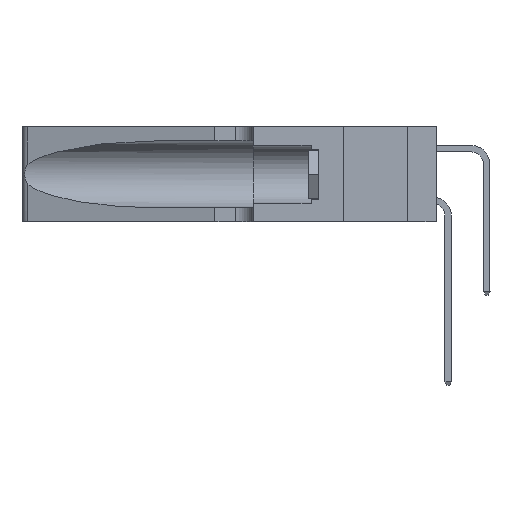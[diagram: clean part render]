
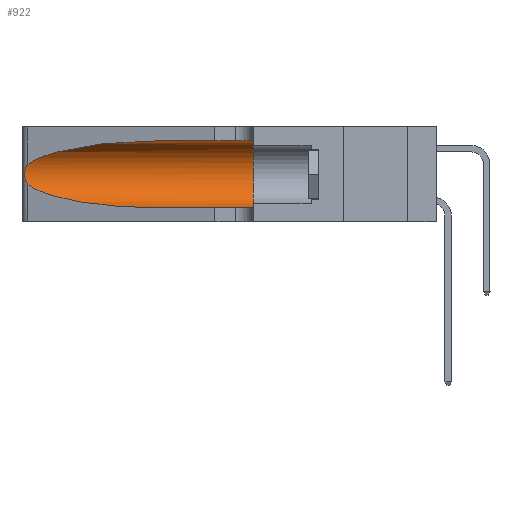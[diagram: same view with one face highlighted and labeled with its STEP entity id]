
A CAD part, left-side view. The second image highlights one B-rep face of the part: STEP entity #922.
In plain terms, the highlighted cylindrical face has radius 3.308 mm (diameter 6.617 mm), a partial arc.
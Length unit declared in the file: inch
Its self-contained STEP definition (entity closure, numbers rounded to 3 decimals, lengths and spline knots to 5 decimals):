
#922 = ADVANCED_FACE ( 'NONE', ( #21679 ), #20278, .F. ) ;
#975 = CARTESIAN_POINT ( 'NONE',  ( 0.25487, 1.22718, 0.14631 ) ) ;
#1325 = AXIS2_PLACEMENT_3D ( 'NONE', #26739, #13287, #20178 ) ;
#2145 = ORIENTED_EDGE ( 'NONE', *, *, #12328, .F. ) ;
#2264 = LINE ( 'NONE', #24805, #27629 ) ;
#3029 = VERTEX_POINT ( 'NONE', #3375 ) ;
#3375 = CARTESIAN_POINT ( 'NONE',  ( 0.1305, 0.35, 0.05475 ) ) ;
#4745 = CARTESIAN_POINT ( 'NONE',  ( 0.25555, 1.22994, 0.2215 ) ) ;
#5323 = CARTESIAN_POINT ( 'NONE',  ( 0.25639, 1.23186, 0.15144 ) ) ;
#6210 = EDGE_LOOP ( 'NONE', ( #10626, #25090, #15269, #28262, #2145, #20049 ) ) ;
#6266 = AXIS2_PLACEMENT_3D ( 'NONE', #13605, #6609, #20293 ) ;
#6609 = DIRECTION ( 'NONE',  ( 0., 1., 0. ) ) ;
#6702 = CIRCLE ( 'NONE', #6266, 0.13025 ) ;
#6811 =( BOUNDED_CURVE ( )  B_SPLINE_CURVE ( 3, ( #16216, #18167, #24859, #27326 ),
 .UNSPECIFIED., .F., .F. ) 
 B_SPLINE_CURVE_WITH_KNOTS ( ( 4, 4 ),
 ( 1.5708, 2.84003 ),
 .UNSPECIFIED. ) 
 CURVE ( )  GEOMETRIC_REPRESENTATION_ITEM ( )  RATIONAL_B_SPLINE_CURVE ( ( 1., 0.87, 0.87, 1. ) ) 
 REPRESENTATION_ITEM ( '' )  );
#7351 = CARTESIAN_POINT ( 'NONE',  ( 0.1305, 0.35, 0.31525 ) ) ;
#9467 = CARTESIAN_POINT ( 'NONE',  ( 0.25487, 1.22718, 0.22369 ) ) ;
#9628 = CARTESIAN_POINT ( 'NONE',  ( 0.26017, 1.23833, 0.17102 ) ) ;
#9807 = EDGE_CURVE ( 'NONE', #10435, #26990, #18684, .T. ) ;
#10435 = VERTEX_POINT ( 'NONE', #19831 ) ;
#10626 = ORIENTED_EDGE ( 'NONE', *, *, #20076, .T. ) ;
#10741 = DIRECTION ( 'NONE',  ( 0., -1., 0. ) ) ;
#10890 = VERTEX_POINT ( 'NONE', #7351 ) ;
#11896 = CARTESIAN_POINT ( 'NONE',  ( 0.25639, 1.23184, 0.21858 ) ) ;
#12328 = EDGE_CURVE ( 'NONE', #10890, #3029, #6702, .T. ) ;
#13084 = VECTOR ( 'NONE', #10741, 39.37008 ) ;
#13287 = DIRECTION ( 'NONE',  ( 0., -1., 0. ) ) ;
#13605 = CARTESIAN_POINT ( 'NONE',  ( 0.1305, 0.35, 0.185 ) ) ;
#13812 = CARTESIAN_POINT ( 'NONE',  ( 0.25487, 1.22718, 0.22369 ) ) ;
#14209 = CARTESIAN_POINT ( 'NONE',  ( 0.25789, 1.23486, 0.15765 ) ) ;
#14402 = CARTESIAN_POINT ( 'NONE',  ( 0.25856, 1.23593, 0.16098 ) ) ;
#14499 = CARTESIAN_POINT ( 'NONE',  ( 0.26075, 1.23896, 0.178 ) ) ;
#14563 = EDGE_CURVE ( 'NONE', #26937, #10890, #2264, .T. ) ;
#14610 = CARTESIAN_POINT ( 'NONE',  ( 0.2373, 1.15595, 0.08982 ) ) ;
#15269 = ORIENTED_EDGE ( 'NONE', *, *, #9807, .T. ) ;
#16216 = CARTESIAN_POINT ( 'NONE',  ( 0.1305, 0.72297, 0.31525 ) ) ;
#16639 = CARTESIAN_POINT ( 'NONE',  ( 0.26075, 1.23896, 0.19203 ) ) ;
#16850 = CARTESIAN_POINT ( 'NONE',  ( 0.1305, 0.72297, 0.05475 ) ) ;
#17880 = CARTESIAN_POINT ( 'NONE',  ( 0.1305, 0.72297, 0.05475 ) ) ;
#18167 = CARTESIAN_POINT ( 'NONE',  ( 0.18966, 0.96281, 0.31525 ) ) ;
#18684 =( BOUNDED_CURVE ( )  B_SPLINE_CURVE ( 3, ( #975, #14610, #25776, #16850 ),
 .UNSPECIFIED., .F., .T. ) 
 B_SPLINE_CURVE_WITH_KNOTS ( ( 4, 4 ),
 ( 3.44316, 4.71239 ),
 .UNSPECIFIED. ) 
 CURVE ( )  GEOMETRIC_REPRESENTATION_ITEM ( )  RATIONAL_B_SPLINE_CURVE ( ( 1., 0.87, 0.87, 1. ) ) 
 REPRESENTATION_ITEM ( '' )  );
#18774 = VERTEX_POINT ( 'NONE', #9467 ) ;
#18793 = CARTESIAN_POINT ( 'NONE',  ( 0.25854, 1.2359, 0.20912 ) ) ;
#19831 = CARTESIAN_POINT ( 'NONE',  ( 0.25487, 1.22718, 0.14631 ) ) ;
#19924 = CARTESIAN_POINT ( 'NONE',  ( 0.1305, 1.61858, 0.05475 ) ) ;
#20049 = ORIENTED_EDGE ( 'NONE', *, *, #14563, .F. ) ;
#20076 = EDGE_CURVE ( 'NONE', #26937, #18774, #6811, .T. ) ;
#20178 = DIRECTION ( 'NONE',  ( 0., 0., -1. ) ) ;
#20278 = CYLINDRICAL_SURFACE ( 'NONE', #1325, 0.13025 ) ;
#20293 = DIRECTION ( 'NONE',  ( 0., 0., 1. ) ) ;
#20480 = LINE ( 'NONE', #19924, #13084 ) ;
#21048 = CARTESIAN_POINT ( 'NONE',  ( 0.25487, 1.22718, 0.14631 ) ) ;
#21679 = FACE_OUTER_BOUND ( 'NONE', #6210, .T. ) ;
#22678 = EDGE_CURVE ( 'NONE', #18774, #10435, #25185, .T. ) ;
#24805 = CARTESIAN_POINT ( 'NONE',  ( 0.1305, 1.61858, 0.31525 ) ) ;
#24859 = CARTESIAN_POINT ( 'NONE',  ( 0.2373, 1.15595, 0.28018 ) ) ;
#25090 = ORIENTED_EDGE ( 'NONE', *, *, #22678, .T. ) ;
#25185 = B_SPLINE_CURVE_WITH_KNOTS ( 'NONE', 3,
 ( #13812, #4745, #11896, #25375, #18793, #27660, #16639, #14499, #9628, #14402, #14209, #5323, #27943, #21048 ),
 .UNSPECIFIED., .F., .F.,
 ( 4, 2, 2, 2, 2, 2, 4 ),
 ( 0., 0.00027, 0.00053, 0.00107, 0.0016, 0.00187, 0.00214 ),
 .UNSPECIFIED. ) ;
#25375 = CARTESIAN_POINT ( 'NONE',  ( 0.25787, 1.23484, 0.2124 ) ) ;
#25776 = CARTESIAN_POINT ( 'NONE',  ( 0.18966, 0.96281, 0.05475 ) ) ;
#26739 = CARTESIAN_POINT ( 'NONE',  ( 0.1305, 1.61858, 0.185 ) ) ;
#26937 = VERTEX_POINT ( 'NONE', #27115 ) ;
#26990 = VERTEX_POINT ( 'NONE', #17880 ) ;
#27050 = DIRECTION ( 'NONE',  ( 0., -1., 0. ) ) ;
#27115 = CARTESIAN_POINT ( 'NONE',  ( 0.1305, 0.72297, 0.31525 ) ) ;
#27326 = CARTESIAN_POINT ( 'NONE',  ( 0.25487, 1.22718, 0.22369 ) ) ;
#27629 = VECTOR ( 'NONE', #27050, 39.37008 ) ;
#27660 = CARTESIAN_POINT ( 'NONE',  ( 0.26018, 1.23835, 0.19895 ) ) ;
#27943 = CARTESIAN_POINT ( 'NONE',  ( 0.25555, 1.22993, 0.14849 ) ) ;
#28262 = ORIENTED_EDGE ( 'NONE', *, *, #28535, .T. ) ;
#28535 = EDGE_CURVE ( 'NONE', #26990, #3029, #20480, .T. ) ;
